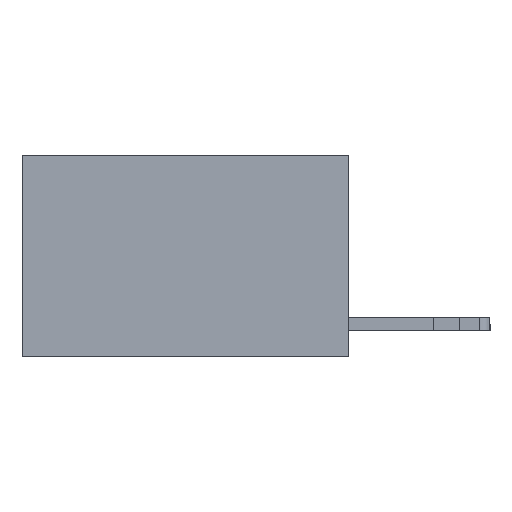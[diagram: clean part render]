
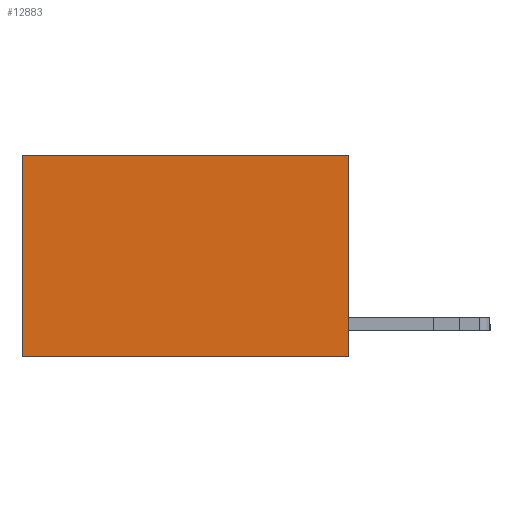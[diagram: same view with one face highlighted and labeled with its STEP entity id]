
A CAD part, left-side view. The second image highlights one B-rep face of the part: STEP entity #12883.
In plain terms, the highlighted planar face has unit normal (-1, 0, 0).
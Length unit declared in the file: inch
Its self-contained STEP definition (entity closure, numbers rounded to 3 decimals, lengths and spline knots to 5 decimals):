
#267 = CARTESIAN_POINT ( 'NONE',  ( 0.2625, 0., 0. ) ) ;
#422 = VERTEX_POINT ( 'NONE', #17207 ) ;
#981 = ORIENTED_EDGE ( 'NONE', *, *, #3301, .F. ) ;
#2219 = DIRECTION ( 'NONE',  ( 0., 0., -1. ) ) ;
#2940 = VECTOR ( 'NONE', #22532, 39.37008 ) ;
#3301 = EDGE_CURVE ( 'NONE', #10517, #422, #22893, .T. ) ;
#3455 = LINE ( 'NONE', #21156, #5994 ) ;
#3903 = PLANE ( 'NONE',  #21504 ) ;
#5065 = EDGE_CURVE ( 'NONE', #7454, #6578, #10658, .T. ) ;
#5994 = VECTOR ( 'NONE', #17279, 39.37008 ) ;
#6578 = VERTEX_POINT ( 'NONE', #11826 ) ;
#7016 = CARTESIAN_POINT ( 'NONE',  ( 0.2625, 0., 0. ) ) ;
#7454 = VERTEX_POINT ( 'NONE', #23709 ) ;
#8372 = EDGE_CURVE ( 'NONE', #10517, #7454, #3455, .T. ) ;
#10223 = VECTOR ( 'NONE', #2219, 39.37008 ) ;
#10517 = VERTEX_POINT ( 'NONE', #20977 ) ;
#10658 = LINE ( 'NONE', #20032, #10223 ) ;
#11826 = CARTESIAN_POINT ( 'NONE',  ( 0.2625, 0.6, -0.37 ) ) ;
#12883 = ADVANCED_FACE ( 'NONE', ( #21748 ), #3903, .F. ) ;
#13019 = DIRECTION ( 'NONE',  ( 0., 0., -1. ) ) ;
#14475 = LINE ( 'NONE', #24489, #2940 ) ;
#14544 = EDGE_LOOP ( 'NONE', ( #24984, #22119, #981, #23612 ) ) ;
#14576 = VECTOR ( 'NONE', #13019, 39.37008 ) ;
#16696 = EDGE_CURVE ( 'NONE', #422, #6578, #14475, .T. ) ;
#17207 = CARTESIAN_POINT ( 'NONE',  ( 0.2625, 0., -0.37 ) ) ;
#17279 = DIRECTION ( 'NONE',  ( 0., 1., 0. ) ) ;
#20032 = CARTESIAN_POINT ( 'NONE',  ( 0.2625, 0.6, 0. ) ) ;
#20977 = CARTESIAN_POINT ( 'NONE',  ( 0.2625, 0., 0. ) ) ;
#21156 = CARTESIAN_POINT ( 'NONE',  ( 0.2625, 0., 0. ) ) ;
#21504 = AXIS2_PLACEMENT_3D ( 'NONE', #267, #24473, #22391 ) ;
#21748 = FACE_OUTER_BOUND ( 'NONE', #14544, .T. ) ;
#22119 = ORIENTED_EDGE ( 'NONE', *, *, #16696, .F. ) ;
#22391 = DIRECTION ( 'NONE',  ( 0., 0., -1. ) ) ;
#22532 = DIRECTION ( 'NONE',  ( 0., 1., 0. ) ) ;
#22893 = LINE ( 'NONE', #7016, #14576 ) ;
#23612 = ORIENTED_EDGE ( 'NONE', *, *, #8372, .T. ) ;
#23709 = CARTESIAN_POINT ( 'NONE',  ( 0.2625, 0.6, 0. ) ) ;
#24473 = DIRECTION ( 'NONE',  ( 1., 0., 0. ) ) ;
#24489 = CARTESIAN_POINT ( 'NONE',  ( 0.2625, 0., -0.37 ) ) ;
#24984 = ORIENTED_EDGE ( 'NONE', *, *, #5065, .T. ) ;
